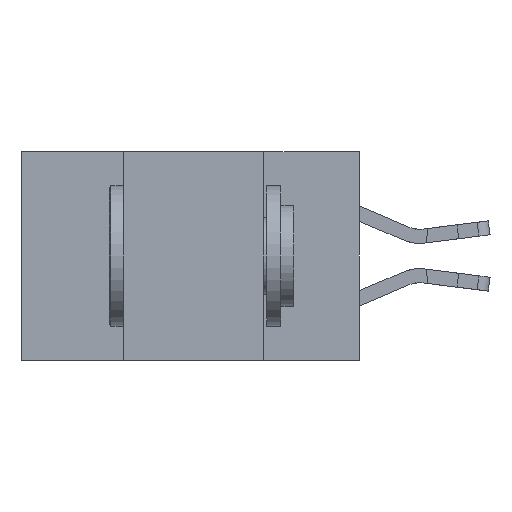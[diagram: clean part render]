
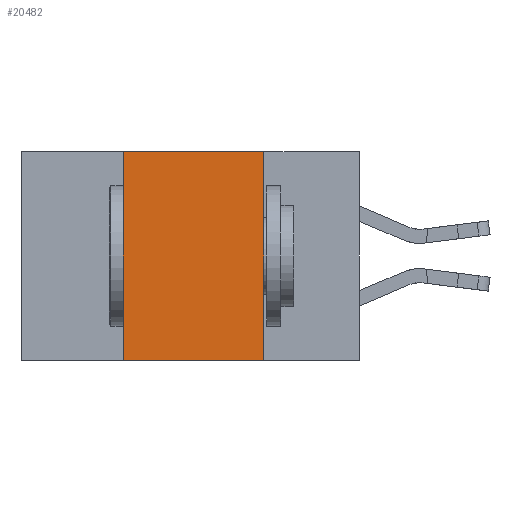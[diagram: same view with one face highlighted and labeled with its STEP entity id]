
A CAD part, left-side view. The second image highlights one B-rep face of the part: STEP entity #20482.
In plain terms, the highlighted planar face has unit normal (-1, 0, 0).
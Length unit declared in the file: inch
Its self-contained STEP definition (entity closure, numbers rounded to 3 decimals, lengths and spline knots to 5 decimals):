
#2108 = LINE ( 'NONE', #4636, #13477 ) ;
#2314 = EDGE_LOOP ( 'NONE', ( #24745, #9832, #10299, #7225 ) ) ;
#4009 = CARTESIAN_POINT ( 'NONE',  ( 0., 0.42, 0. ) ) ;
#4337 = CARTESIAN_POINT ( 'NONE',  ( 0., 0.6, 0. ) ) ;
#4636 = CARTESIAN_POINT ( 'NONE',  ( 0., 0.17, 0. ) ) ;
#5521 = EDGE_CURVE ( 'NONE', #7793, #20075, #24161, .T. ) ;
#6210 = CARTESIAN_POINT ( 'NONE',  ( 0., 0.17, 0. ) ) ;
#6700 = VECTOR ( 'NONE', #19615, 39.37008 ) ;
#7225 = ORIENTED_EDGE ( 'NONE', *, *, #15307, .T. ) ;
#7631 = LINE ( 'NONE', #9158, #6700 ) ;
#7723 = VECTOR ( 'NONE', #8064, 39.37008 ) ;
#7793 = VERTEX_POINT ( 'NONE', #24627 ) ;
#8064 = DIRECTION ( 'NONE',  ( 0., 0., 1. ) ) ;
#9158 = CARTESIAN_POINT ( 'NONE',  ( 0., 0.6, -0.37 ) ) ;
#9532 = DIRECTION ( 'NONE',  ( 0., -1., 0. ) ) ;
#9832 = ORIENTED_EDGE ( 'NONE', *, *, #15713, .F. ) ;
#10051 = DIRECTION ( 'NONE',  ( 1., 0., 0. ) ) ;
#10299 = ORIENTED_EDGE ( 'NONE', *, *, #5521, .F. ) ;
#10405 = VECTOR ( 'NONE', #9532, 39.37008 ) ;
#10938 = FACE_OUTER_BOUND ( 'NONE', #2314, .T. ) ;
#12582 = CARTESIAN_POINT ( 'NONE',  ( 0., 0.17, -0.37 ) ) ;
#13477 = VECTOR ( 'NONE', #20534, 39.37008 ) ;
#14668 = CARTESIAN_POINT ( 'NONE',  ( 0., 0.42, 0. ) ) ;
#15307 = EDGE_CURVE ( 'NONE', #7793, #25527, #7631, .T. ) ;
#15574 = EDGE_CURVE ( 'NONE', #17951, #25527, #2108, .T. ) ;
#15713 = EDGE_CURVE ( 'NONE', #20075, #17951, #24379, .T. ) ;
#17951 = VERTEX_POINT ( 'NONE', #6210 ) ;
#19615 = DIRECTION ( 'NONE',  ( 0., -1., 0. ) ) ;
#20075 = VERTEX_POINT ( 'NONE', #14668 ) ;
#20148 = PLANE ( 'NONE',  #23820 ) ;
#20482 = ADVANCED_FACE ( 'NONE', ( #10938 ), #20148, .F. ) ;
#20534 = DIRECTION ( 'NONE',  ( 0., 0., -1. ) ) ;
#21387 = CARTESIAN_POINT ( 'NONE',  ( 0., 0.6, 0. ) ) ;
#21907 = DIRECTION ( 'NONE',  ( 0., 0., -1. ) ) ;
#23820 = AXIS2_PLACEMENT_3D ( 'NONE', #4337, #10051, #21907 ) ;
#24161 = LINE ( 'NONE', #4009, #7723 ) ;
#24379 = LINE ( 'NONE', #21387, #10405 ) ;
#24627 = CARTESIAN_POINT ( 'NONE',  ( 0., 0.42, -0.37 ) ) ;
#24745 = ORIENTED_EDGE ( 'NONE', *, *, #15574, .F. ) ;
#25527 = VERTEX_POINT ( 'NONE', #12582 ) ;
